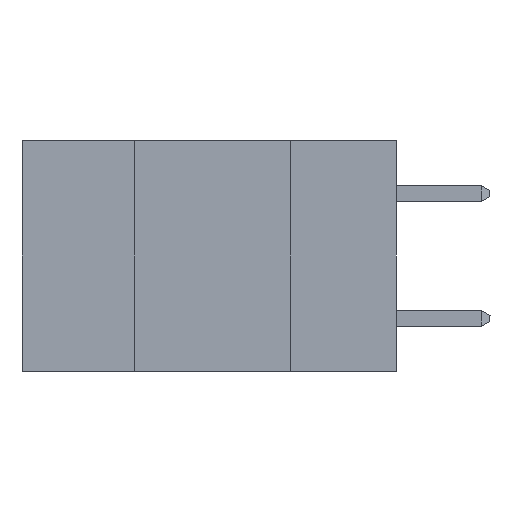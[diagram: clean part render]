
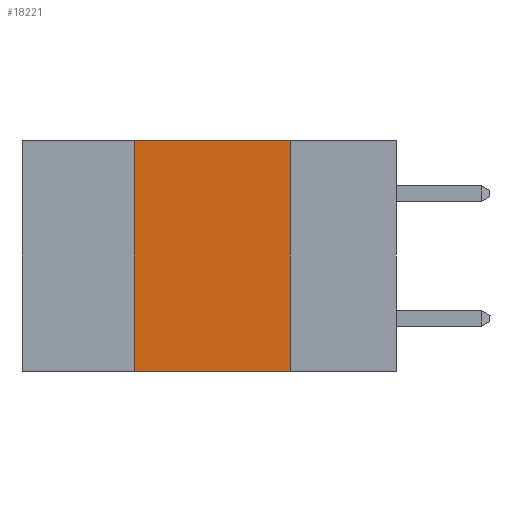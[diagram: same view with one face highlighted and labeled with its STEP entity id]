
A CAD part, left-side view. The second image highlights one B-rep face of the part: STEP entity #18221.
In plain terms, the highlighted planar face has unit normal (-1, 0, 0).
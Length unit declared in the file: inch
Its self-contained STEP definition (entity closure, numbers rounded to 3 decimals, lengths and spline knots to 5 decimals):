
#17 = DIRECTION ( 'NONE',  ( 0., 0., 1. ) ) ;
#1619 = CARTESIAN_POINT ( 'NONE',  ( 0., 0.42, 0. ) ) ;
#2318 = DIRECTION ( 'NONE',  ( 0., -1., 0. ) ) ;
#2810 = LINE ( 'NONE', #8464, #16627 ) ;
#3938 = CARTESIAN_POINT ( 'NONE',  ( 0., 0.6, -0.37 ) ) ;
#4087 = CARTESIAN_POINT ( 'NONE',  ( 0., 0.17, 0. ) ) ;
#4579 = EDGE_LOOP ( 'NONE', ( #14167, #7863, #16632, #16769 ) ) ;
#4668 = AXIS2_PLACEMENT_3D ( 'NONE', #11171, #14306, #4820 ) ;
#4820 = DIRECTION ( 'NONE',  ( 0., 0., -1. ) ) ;
#4964 = CARTESIAN_POINT ( 'NONE',  ( 0., 0.42, 0. ) ) ;
#5112 = EDGE_CURVE ( 'NONE', #17467, #15679, #16686, .T. ) ;
#5365 = LINE ( 'NONE', #3938, #5850 ) ;
#5537 = CARTESIAN_POINT ( 'NONE',  ( 0., 0.6, 0. ) ) ;
#5850 = VECTOR ( 'NONE', #2318, 39.37008 ) ;
#6280 = PLANE ( 'NONE',  #4668 ) ;
#7863 = ORIENTED_EDGE ( 'NONE', *, *, #14861, .F. ) ;
#8093 = VERTEX_POINT ( 'NONE', #4087 ) ;
#8158 = CARTESIAN_POINT ( 'NONE',  ( 0., 0.17, -0.37 ) ) ;
#8464 = CARTESIAN_POINT ( 'NONE',  ( 0., 0.17, 0. ) ) ;
#8885 = EDGE_CURVE ( 'NONE', #8093, #19620, #2810, .T. ) ;
#11171 = CARTESIAN_POINT ( 'NONE',  ( 0., 0.6, 0. ) ) ;
#12530 = CARTESIAN_POINT ( 'NONE',  ( 0., 0.42, -0.37 ) ) ;
#12655 = EDGE_CURVE ( 'NONE', #17467, #19620, #5365, .T. ) ;
#14167 = ORIENTED_EDGE ( 'NONE', *, *, #8885, .F. ) ;
#14306 = DIRECTION ( 'NONE',  ( 1., 0., 0. ) ) ;
#14861 = EDGE_CURVE ( 'NONE', #15679, #8093, #14935, .T. ) ;
#14935 = LINE ( 'NONE', #5537, #17637 ) ;
#15178 = DIRECTION ( 'NONE',  ( 0., -1., 0. ) ) ;
#15540 = FACE_OUTER_BOUND ( 'NONE', #4579, .T. ) ;
#15679 = VERTEX_POINT ( 'NONE', #1619 ) ;
#16211 = VECTOR ( 'NONE', #17, 39.37008 ) ;
#16627 = VECTOR ( 'NONE', #19767, 39.37008 ) ;
#16632 = ORIENTED_EDGE ( 'NONE', *, *, #5112, .F. ) ;
#16686 = LINE ( 'NONE', #4964, #16211 ) ;
#16769 = ORIENTED_EDGE ( 'NONE', *, *, #12655, .T. ) ;
#17467 = VERTEX_POINT ( 'NONE', #12530 ) ;
#17637 = VECTOR ( 'NONE', #15178, 39.37008 ) ;
#18221 = ADVANCED_FACE ( 'NONE', ( #15540 ), #6280, .F. ) ;
#19620 = VERTEX_POINT ( 'NONE', #8158 ) ;
#19767 = DIRECTION ( 'NONE',  ( 0., 0., -1. ) ) ;
